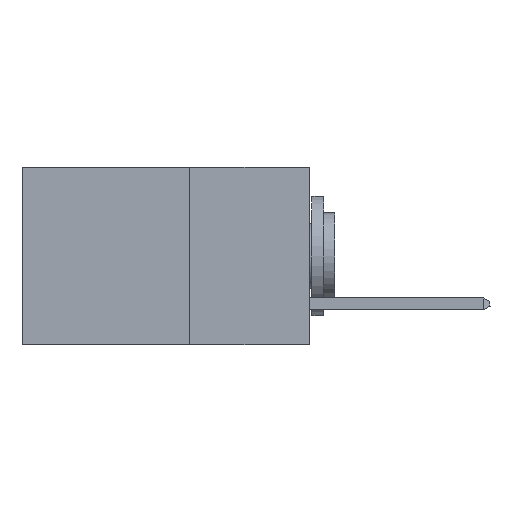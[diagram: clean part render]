
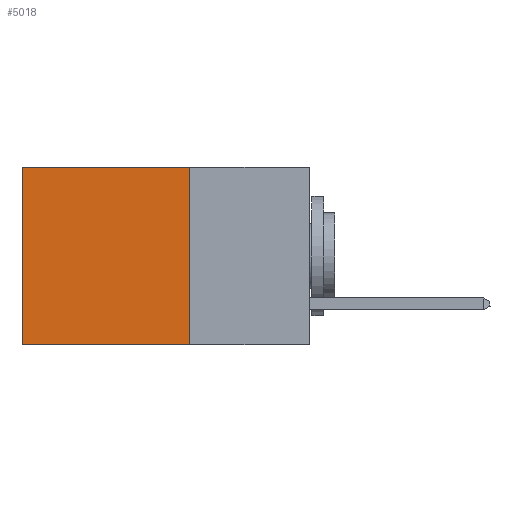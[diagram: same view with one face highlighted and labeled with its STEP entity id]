
A CAD part, left-side view. The second image highlights one B-rep face of the part: STEP entity #5018.
In plain terms, the highlighted planar face has unit normal (-1, 0, 0).
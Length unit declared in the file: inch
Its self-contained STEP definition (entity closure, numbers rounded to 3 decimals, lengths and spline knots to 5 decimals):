
#28 = ORIENTED_EDGE ( 'NONE', *, *, #20213, .T. ) ;
#55 = PLANE ( 'NONE',  #22516 ) ;
#531 = VERTEX_POINT ( 'NONE', #2271 ) ;
#662 = CARTESIAN_POINT ( 'NONE',  ( 0.2875, 0.25, -0.37 ) ) ;
#1336 = CARTESIAN_POINT ( 'NONE',  ( 0.2875, 0.25, -0.37 ) ) ;
#2271 = CARTESIAN_POINT ( 'NONE',  ( 0.2875, 0.6, 0. ) ) ;
#4593 = CARTESIAN_POINT ( 'NONE',  ( 0.2875, 0.25, 0. ) ) ;
#5018 = ADVANCED_FACE ( 'NONE', ( #19685 ), #55, .F. ) ;
#5470 = LINE ( 'NONE', #1336, #31821 ) ;
#7113 = VECTOR ( 'NONE', #26366, 39.37008 ) ;
#7234 = DIRECTION ( 'NONE',  ( 0., 1., 0. ) ) ;
#7886 = VERTEX_POINT ( 'NONE', #19863 ) ;
#9978 = LINE ( 'NONE', #35567, #34821 ) ;
#10060 = LINE ( 'NONE', #23375, #7113 ) ;
#10846 = EDGE_CURVE ( 'NONE', #7886, #20391, #26119, .T. ) ;
#12053 = EDGE_CURVE ( 'NONE', #20391, #30662, #5470, .T. ) ;
#13440 = VECTOR ( 'NONE', #38602, 39.37008 ) ;
#14160 = DIRECTION ( 'NONE',  ( 0., 1., 0. ) ) ;
#15873 = DIRECTION ( 'NONE',  ( 0., 0., -1. ) ) ;
#17527 = CARTESIAN_POINT ( 'NONE',  ( 0.2875, 0.6, -0.37 ) ) ;
#19685 = FACE_OUTER_BOUND ( 'NONE', #39837, .T. ) ;
#19863 = CARTESIAN_POINT ( 'NONE',  ( 0.2875, 0.25, 0. ) ) ;
#20213 = EDGE_CURVE ( 'NONE', #7886, #531, #9978, .T. ) ;
#20391 = VERTEX_POINT ( 'NONE', #662 ) ;
#22516 = AXIS2_PLACEMENT_3D ( 'NONE', #34506, #40290, #15873 ) ;
#23375 = CARTESIAN_POINT ( 'NONE',  ( 0.2875, 0.6, 0. ) ) ;
#24695 = ORIENTED_EDGE ( 'NONE', *, *, #12053, .F. ) ;
#26119 = LINE ( 'NONE', #4593, #13440 ) ;
#26366 = DIRECTION ( 'NONE',  ( 0., 0., -1. ) ) ;
#27939 = ORIENTED_EDGE ( 'NONE', *, *, #10846, .F. ) ;
#30662 = VERTEX_POINT ( 'NONE', #17527 ) ;
#31821 = VECTOR ( 'NONE', #14160, 39.37008 ) ;
#34506 = CARTESIAN_POINT ( 'NONE',  ( 0.2875, 0.25, 0. ) ) ;
#34821 = VECTOR ( 'NONE', #7234, 39.37008 ) ;
#35567 = CARTESIAN_POINT ( 'NONE',  ( 0.2875, 0.25, 0. ) ) ;
#38602 = DIRECTION ( 'NONE',  ( 0., 0., -1. ) ) ;
#39615 = ORIENTED_EDGE ( 'NONE', *, *, #39767, .T. ) ;
#39767 = EDGE_CURVE ( 'NONE', #531, #30662, #10060, .T. ) ;
#39837 = EDGE_LOOP ( 'NONE', ( #39615, #24695, #27939, #28 ) ) ;
#40290 = DIRECTION ( 'NONE',  ( 1., 0., 0. ) ) ;
